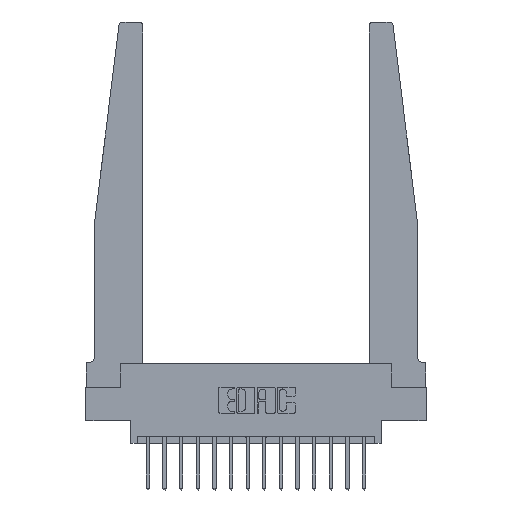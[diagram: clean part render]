
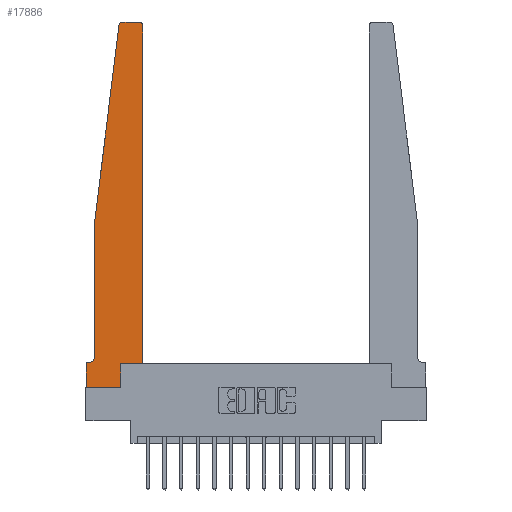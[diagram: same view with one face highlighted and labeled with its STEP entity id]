
A CAD part, top view. The second image highlights one B-rep face of the part: STEP entity #17886.
In plain terms, the highlighted planar face has unit normal (0, 0, 1).
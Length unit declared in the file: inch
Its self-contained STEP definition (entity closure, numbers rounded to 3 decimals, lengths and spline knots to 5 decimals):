
#345 = VERTEX_POINT ( 'NONE', #1629 ) ;
#384 = DIRECTION ( 'NONE',  ( 0., 0., 1. ) ) ;
#480 = CARTESIAN_POINT ( 'NONE',  ( 0., 0.1875, 0.37 ) ) ;
#493 = LINE ( 'NONE', #1791, #12019 ) ;
#1064 = CARTESIAN_POINT ( 'NONE',  ( 0.425, 0.18, 0.37 ) ) ;
#1104 = LINE ( 'NONE', #13726, #7996 ) ;
#1276 = DIRECTION ( 'NONE',  ( 1., 0., 0. ) ) ;
#1284 = EDGE_CURVE ( 'NONE', #4956, #7516, #10437, .T. ) ;
#1450 = VECTOR ( 'NONE', #4597, 39.37008 ) ;
#1629 = CARTESIAN_POINT ( 'NONE',  ( 0.27653, 2.75, 0.37 ) ) ;
#1791 = CARTESIAN_POINT ( 'NONE',  ( 0.065, 1.25, 0.37 ) ) ;
#1907 = CARTESIAN_POINT ( 'NONE',  ( 0.425, 2.72, 0.37 ) ) ;
#2005 = CARTESIAN_POINT ( 'NONE',  ( 0.2605, 0.18, 0.37 ) ) ;
#2073 = EDGE_CURVE ( 'NONE', #16875, #12993, #1104, .T. ) ;
#2416 = EDGE_CURVE ( 'NONE', #6445, #345, #11341, .T. ) ;
#2592 = VECTOR ( 'NONE', #10814, 39.37008 ) ;
#2971 = DIRECTION ( 'NONE',  ( -1., 0., 0. ) ) ;
#3006 = CARTESIAN_POINT ( 'NONE',  ( 0.065, 1.25, 0.37 ) ) ;
#3399 = VERTEX_POINT ( 'NONE', #11289 ) ;
#3577 = VERTEX_POINT ( 'NONE', #17874 ) ;
#3971 = VERTEX_POINT ( 'NONE', #10313 ) ;
#4299 = CARTESIAN_POINT ( 'NONE',  ( 0., 0.1875, 0.37 ) ) ;
#4338 = CIRCLE ( 'NONE', #6387, 0.03 ) ;
#4352 = DIRECTION ( 'NONE',  ( 0., -1., 0. ) ) ;
#4492 = DIRECTION ( 'NONE',  ( 1., 0., 0. ) ) ;
#4597 = DIRECTION ( 'NONE',  ( 0., 1., 0. ) ) ;
#4709 = CARTESIAN_POINT ( 'NONE',  ( 0., 0., 0.37 ) ) ;
#4956 = VERTEX_POINT ( 'NONE', #1064 ) ;
#5089 = CARTESIAN_POINT ( 'NONE',  ( 0.395, 2.72, 0.37 ) ) ;
#5276 = DIRECTION ( 'NONE',  ( 1., 0., 0. ) ) ;
#5308 = ORIENTED_EDGE ( 'NONE', *, *, #12072, .T. ) ;
#5461 = CARTESIAN_POINT ( 'NONE',  ( 0.27653, 2.72, 0.37 ) ) ;
#5852 = CIRCLE ( 'NONE', #8256, 0.05 ) ;
#5934 = VECTOR ( 'NONE', #4352, 39.37008 ) ;
#5969 = FACE_OUTER_BOUND ( 'NONE', #14011, .T. ) ;
#6005 = LINE ( 'NONE', #4709, #17517 ) ;
#6088 = DIRECTION ( 'NONE',  ( 1., 0., 0. ) ) ;
#6100 = VERTEX_POINT ( 'NONE', #7766 ) ;
#6138 = AXIS2_PLACEMENT_3D ( 'NONE', #5089, #10741, #5276 ) ;
#6387 = AXIS2_PLACEMENT_3D ( 'NONE', #5461, #14003, #1276 ) ;
#6445 = VERTEX_POINT ( 'NONE', #15711 ) ;
#6669 = ORIENTED_EDGE ( 'NONE', *, *, #8851, .T. ) ;
#6773 = ORIENTED_EDGE ( 'NONE', *, *, #11142, .T. ) ;
#6818 = LINE ( 'NONE', #9973, #16089 ) ;
#7516 = VERTEX_POINT ( 'NONE', #1907 ) ;
#7542 = CARTESIAN_POINT ( 'NONE',  ( 0.24675, 2.72367, 0.37 ) ) ;
#7766 = CARTESIAN_POINT ( 'NONE',  ( 0.065, 1.25, 0.37 ) ) ;
#7867 = VECTOR ( 'NONE', #2971, 39.37008 ) ;
#7996 = VECTOR ( 'NONE', #10754, 39.37008 ) ;
#8256 = AXIS2_PLACEMENT_3D ( 'NONE', #16180, #14803, #10538 ) ;
#8851 = EDGE_CURVE ( 'NONE', #345, #9601, #4338, .T. ) ;
#8855 = PLANE ( 'NONE',  #16724 ) ;
#9235 = EDGE_CURVE ( 'NONE', #9601, #6100, #493, .T. ) ;
#9601 = VERTEX_POINT ( 'NONE', #7542 ) ;
#9973 = CARTESIAN_POINT ( 'NONE',  ( 0., 0., 0.37 ) ) ;
#10313 = CARTESIAN_POINT ( 'NONE',  ( 0., 0., 0.37 ) ) ;
#10437 = LINE ( 'NONE', #11728, #1450 ) ;
#10538 = DIRECTION ( 'NONE',  ( -1., 0., 0. ) ) ;
#10601 = VECTOR ( 'NONE', #6088, 39.37008 ) ;
#10741 = DIRECTION ( 'NONE',  ( 0., 0., 1. ) ) ;
#10754 = DIRECTION ( 'NONE',  ( -1., 0., 0. ) ) ;
#10814 = DIRECTION ( 'NONE',  ( 0., 1., 0. ) ) ;
#11142 = EDGE_CURVE ( 'NONE', #16173, #3577, #14705, .T. ) ;
#11289 = CARTESIAN_POINT ( 'NONE',  ( 0.065, 0.2375, 0.37 ) ) ;
#11341 = LINE ( 'NONE', #11430, #7867 ) ;
#11361 = CARTESIAN_POINT ( 'NONE',  ( 0.2605, 0., 0.37 ) ) ;
#11430 = CARTESIAN_POINT ( 'NONE',  ( 0.25, 2.75, 0.37 ) ) ;
#11728 = CARTESIAN_POINT ( 'NONE',  ( 0.425, 0.18, 0.37 ) ) ;
#12019 = VECTOR ( 'NONE', #15802, 39.37008 ) ;
#12072 = EDGE_CURVE ( 'NONE', #7516, #6445, #15624, .T. ) ;
#12250 = ORIENTED_EDGE ( 'NONE', *, *, #12387, .T. ) ;
#12308 = EDGE_CURVE ( 'NONE', #3577, #4956, #15816, .T. ) ;
#12387 = EDGE_CURVE ( 'NONE', #3399, #16875, #5852, .T. ) ;
#12545 = ORIENTED_EDGE ( 'NONE', *, *, #16540, .T. ) ;
#12565 = ORIENTED_EDGE ( 'NONE', *, *, #9235, .T. ) ;
#12618 = ORIENTED_EDGE ( 'NONE', *, *, #2416, .T. ) ;
#12993 = VERTEX_POINT ( 'NONE', #4299 ) ;
#13121 = CARTESIAN_POINT ( 'NONE',  ( 0.425, 0.18, 0.37 ) ) ;
#13572 = EDGE_CURVE ( 'NONE', #6100, #3399, #15737, .T. ) ;
#13621 = ORIENTED_EDGE ( 'NONE', *, *, #14817, .T. ) ;
#13726 = CARTESIAN_POINT ( 'NONE',  ( 0.065, 0.1875, 0.37 ) ) ;
#13952 = CARTESIAN_POINT ( 'NONE',  ( 0.015, 0.1875, 0.37 ) ) ;
#14003 = DIRECTION ( 'NONE',  ( 0., 0., 1. ) ) ;
#14011 = EDGE_LOOP ( 'NONE', ( #12618, #6669, #12565, #16341, #12250, #16002, #12545, #13621, #6773, #14526, #14757, #5308 ) ) ;
#14158 = DIRECTION ( 'NONE',  ( 0., -1., 0. ) ) ;
#14526 = ORIENTED_EDGE ( 'NONE', *, *, #12308, .T. ) ;
#14705 = LINE ( 'NONE', #2005, #2592 ) ;
#14757 = ORIENTED_EDGE ( 'NONE', *, *, #1284, .T. ) ;
#14803 = DIRECTION ( 'NONE',  ( 0., 0., -1. ) ) ;
#14817 = EDGE_CURVE ( 'NONE', #3971, #16173, #6005, .T. ) ;
#15624 = CIRCLE ( 'NONE', #6138, 0.03 ) ;
#15711 = CARTESIAN_POINT ( 'NONE',  ( 0.395, 2.75, 0.37 ) ) ;
#15737 = LINE ( 'NONE', #3006, #5934 ) ;
#15802 = DIRECTION ( 'NONE',  ( -0.122, -0.992, 0. ) ) ;
#15816 = LINE ( 'NONE', #13121, #10601 ) ;
#16002 = ORIENTED_EDGE ( 'NONE', *, *, #2073, .T. ) ;
#16089 = VECTOR ( 'NONE', #14158, 39.37008 ) ;
#16173 = VERTEX_POINT ( 'NONE', #11361 ) ;
#16180 = CARTESIAN_POINT ( 'NONE',  ( 0.015, 0.2375, 0.37 ) ) ;
#16341 = ORIENTED_EDGE ( 'NONE', *, *, #13572, .T. ) ;
#16540 = EDGE_CURVE ( 'NONE', #12993, #3971, #6818, .T. ) ;
#16724 = AXIS2_PLACEMENT_3D ( 'NONE', #480, #384, #4492 ) ;
#16875 = VERTEX_POINT ( 'NONE', #13952 ) ;
#17258 = DIRECTION ( 'NONE',  ( 1., 0., 0. ) ) ;
#17517 = VECTOR ( 'NONE', #17258, 39.37008 ) ;
#17874 = CARTESIAN_POINT ( 'NONE',  ( 0.2605, 0.18, 0.37 ) ) ;
#17886 = ADVANCED_FACE ( 'NONE', ( #5969 ), #8855, .T. ) ;
